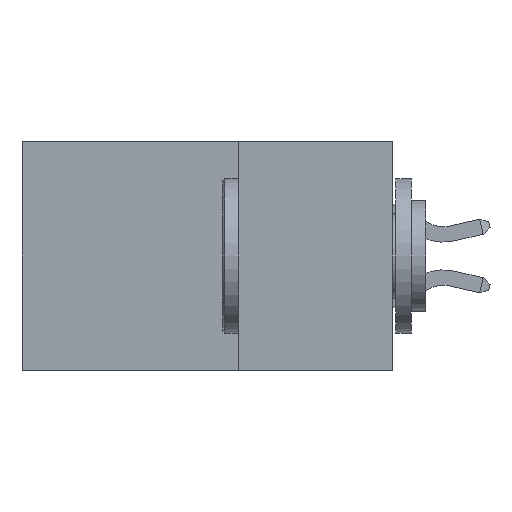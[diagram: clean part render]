
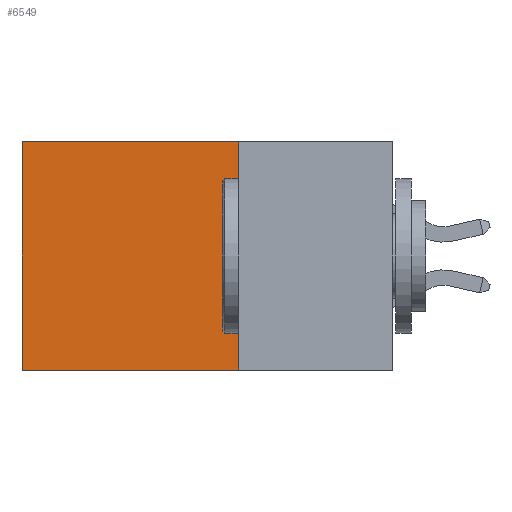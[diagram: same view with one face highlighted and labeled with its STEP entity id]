
A CAD part, left-side view. The second image highlights one B-rep face of the part: STEP entity #6549.
In plain terms, the highlighted planar face has unit normal (-1, 0, 0).
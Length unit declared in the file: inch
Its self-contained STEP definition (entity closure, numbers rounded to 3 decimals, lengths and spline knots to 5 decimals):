
#662 = LINE ( 'NONE', #2382, #8083 ) ;
#769 = PLANE ( 'NONE',  #8887 ) ;
#1293 = CARTESIAN_POINT ( 'NONE',  ( 0.2875, 0.25, -0.37 ) ) ;
#1630 = LINE ( 'NONE', #2522, #15085 ) ;
#2215 = DIRECTION ( 'NONE',  ( 1., 0., 0. ) ) ;
#2382 = CARTESIAN_POINT ( 'NONE',  ( 0.2875, 0.25, 0. ) ) ;
#2424 = ORIENTED_EDGE ( 'NONE', *, *, #4756, .T. ) ;
#2522 = CARTESIAN_POINT ( 'NONE',  ( 0.2875, 0.25, 0. ) ) ;
#3623 = VECTOR ( 'NONE', #10744, 39.37008 ) ;
#4756 = EDGE_CURVE ( 'NONE', #9386, #16262, #1630, .T. ) ;
#5021 = CARTESIAN_POINT ( 'NONE',  ( 0.2875, 0.6, 0. ) ) ;
#5589 = FACE_OUTER_BOUND ( 'NONE', #15068, .T. ) ;
#6049 = ORIENTED_EDGE ( 'NONE', *, *, #14758, .T. ) ;
#6365 = DIRECTION ( 'NONE',  ( 0., 0., -1. ) ) ;
#6549 = ADVANCED_FACE ( 'NONE', ( #5589 ), #769, .F. ) ;
#7118 = VECTOR ( 'NONE', #6365, 39.37008 ) ;
#7235 = VERTEX_POINT ( 'NONE', #15127 ) ;
#7321 = EDGE_CURVE ( 'NONE', #9386, #7235, #662, .T. ) ;
#8083 = VECTOR ( 'NONE', #11669, 39.37008 ) ;
#8887 = AXIS2_PLACEMENT_3D ( 'NONE', #16404, #2215, #11526 ) ;
#9386 = VERTEX_POINT ( 'NONE', #12979 ) ;
#9678 = ORIENTED_EDGE ( 'NONE', *, *, #7321, .F. ) ;
#10518 = LINE ( 'NONE', #5021, #7118 ) ;
#10599 = ORIENTED_EDGE ( 'NONE', *, *, #11641, .F. ) ;
#10744 = DIRECTION ( 'NONE',  ( 0., 1., 0. ) ) ;
#11526 = DIRECTION ( 'NONE',  ( 0., 0., -1. ) ) ;
#11641 = EDGE_CURVE ( 'NONE', #7235, #14445, #12764, .T. ) ;
#11669 = DIRECTION ( 'NONE',  ( 0., 0., -1. ) ) ;
#11787 = DIRECTION ( 'NONE',  ( 0., 1., 0. ) ) ;
#11894 = CARTESIAN_POINT ( 'NONE',  ( 0.2875, 0.6, -0.37 ) ) ;
#12764 = LINE ( 'NONE', #1293, #3623 ) ;
#12979 = CARTESIAN_POINT ( 'NONE',  ( 0.2875, 0.25, 0. ) ) ;
#14445 = VERTEX_POINT ( 'NONE', #11894 ) ;
#14758 = EDGE_CURVE ( 'NONE', #16262, #14445, #10518, .T. ) ;
#15068 = EDGE_LOOP ( 'NONE', ( #6049, #10599, #9678, #2424 ) ) ;
#15085 = VECTOR ( 'NONE', #11787, 39.37008 ) ;
#15127 = CARTESIAN_POINT ( 'NONE',  ( 0.2875, 0.25, -0.37 ) ) ;
#16262 = VERTEX_POINT ( 'NONE', #16884 ) ;
#16404 = CARTESIAN_POINT ( 'NONE',  ( 0.2875, 0.25, 0. ) ) ;
#16884 = CARTESIAN_POINT ( 'NONE',  ( 0.2875, 0.6, 0. ) ) ;
